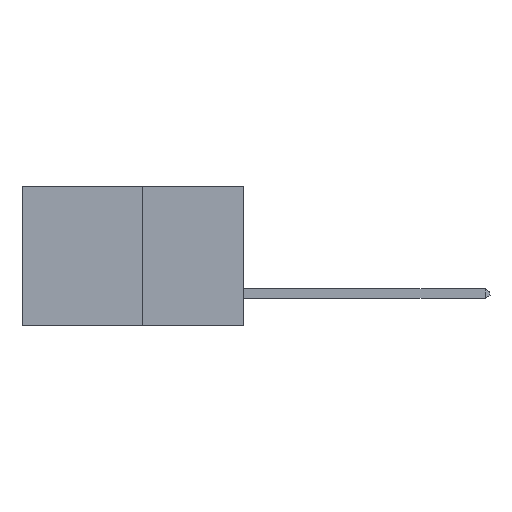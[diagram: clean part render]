
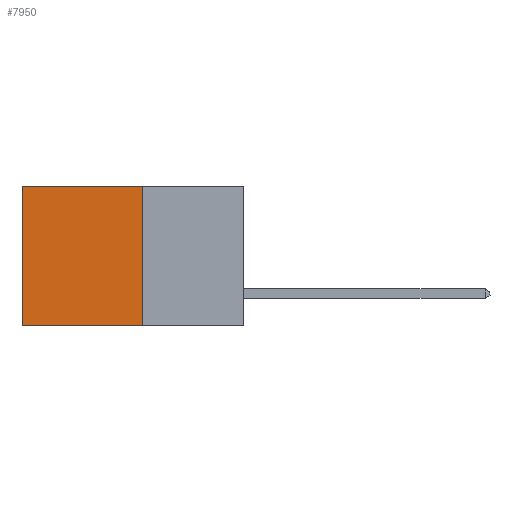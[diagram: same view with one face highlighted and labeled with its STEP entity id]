
A CAD part, left-side view. The second image highlights one B-rep face of the part: STEP entity #7950.
In plain terms, the highlighted planar face has unit normal (-1, 0, 0).
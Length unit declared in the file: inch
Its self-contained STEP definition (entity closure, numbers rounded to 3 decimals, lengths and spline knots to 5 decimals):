
#65 = ORIENTED_EDGE ( 'NONE', *, *, #5867, .F. ) ;
#2058 = ORIENTED_EDGE ( 'NONE', *, *, #8218, .T. ) ;
#2167 = DIRECTION ( 'NONE',  ( 1., 0., 0. ) ) ;
#2680 = LINE ( 'NONE', #6365, #5033 ) ;
#2988 = EDGE_CURVE ( 'NONE', #6072, #6777, #11481, .T. ) ;
#3215 = VERTEX_POINT ( 'NONE', #7310 ) ;
#3369 = ORIENTED_EDGE ( 'NONE', *, *, #6085, .F. ) ;
#3797 = DIRECTION ( 'NONE',  ( 0., 0., -1. ) ) ;
#4454 = AXIS2_PLACEMENT_3D ( 'NONE', #8082, #2167, #9081 ) ;
#4826 = CARTESIAN_POINT ( 'NONE',  ( 0.277, 0.27, 0. ) ) ;
#5033 = VECTOR ( 'NONE', #10150, 39.37008 ) ;
#5791 = VECTOR ( 'NONE', #6062, 39.37008 ) ;
#5867 = EDGE_CURVE ( 'NONE', #5968, #3215, #6400, .T. ) ;
#5968 = VERTEX_POINT ( 'NONE', #8085 ) ;
#6062 = DIRECTION ( 'NONE',  ( 0., 0., -1. ) ) ;
#6072 = VERTEX_POINT ( 'NONE', #7271 ) ;
#6085 = EDGE_CURVE ( 'NONE', #3215, #6777, #2680, .T. ) ;
#6308 = CARTESIAN_POINT ( 'NONE',  ( 0.277, 0.59, -0.37 ) ) ;
#6365 = CARTESIAN_POINT ( 'NONE',  ( 0.277, 0.27, -0.37 ) ) ;
#6400 = LINE ( 'NONE', #11696, #5791 ) ;
#6777 = VERTEX_POINT ( 'NONE', #6308 ) ;
#7041 = EDGE_LOOP ( 'NONE', ( #12126, #3369, #65, #2058 ) ) ;
#7271 = CARTESIAN_POINT ( 'NONE',  ( 0.277, 0.59, 0. ) ) ;
#7310 = CARTESIAN_POINT ( 'NONE',  ( 0.277, 0.27, -0.37 ) ) ;
#7950 = ADVANCED_FACE ( 'NONE', ( #10516 ), #10901, .F. ) ;
#8082 = CARTESIAN_POINT ( 'NONE',  ( 0.277, 0.27, -0.37 ) ) ;
#8085 = CARTESIAN_POINT ( 'NONE',  ( 0.277, 0.27, 0. ) ) ;
#8218 = EDGE_CURVE ( 'NONE', #5968, #6072, #10091, .T. ) ;
#9058 = VECTOR ( 'NONE', #3797, 39.37008 ) ;
#9081 = DIRECTION ( 'NONE',  ( 0., 0., -1. ) ) ;
#9654 = DIRECTION ( 'NONE',  ( 0., 1., 0. ) ) ;
#10091 = LINE ( 'NONE', #4826, #12144 ) ;
#10150 = DIRECTION ( 'NONE',  ( 0., 1., 0. ) ) ;
#10516 = FACE_OUTER_BOUND ( 'NONE', #7041, .T. ) ;
#10901 = PLANE ( 'NONE',  #4454 ) ;
#11481 = LINE ( 'NONE', #12472, #9058 ) ;
#11696 = CARTESIAN_POINT ( 'NONE',  ( 0.277, 0.27, -0.37 ) ) ;
#12126 = ORIENTED_EDGE ( 'NONE', *, *, #2988, .T. ) ;
#12144 = VECTOR ( 'NONE', #9654, 39.37008 ) ;
#12472 = CARTESIAN_POINT ( 'NONE',  ( 0.277, 0.59, -0.37 ) ) ;
